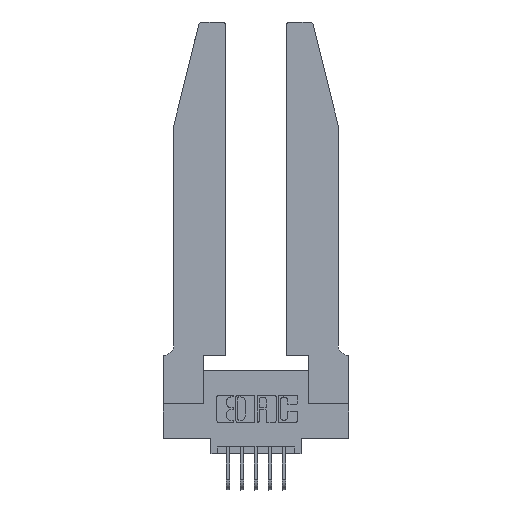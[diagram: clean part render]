
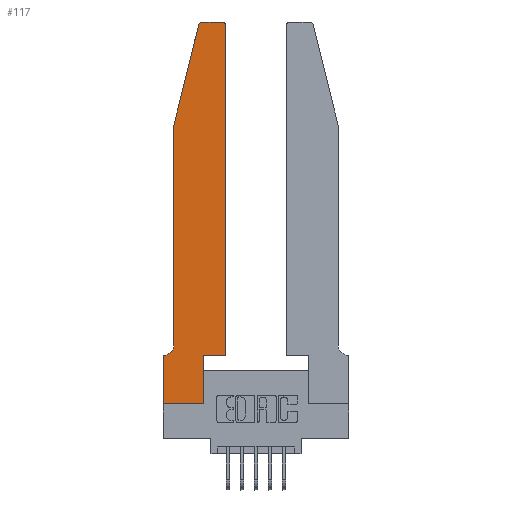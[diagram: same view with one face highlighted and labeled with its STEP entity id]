
A CAD part, top view. The second image highlights one B-rep face of the part: STEP entity #117.
In plain terms, the highlighted planar face has unit normal (0, 0, 1).
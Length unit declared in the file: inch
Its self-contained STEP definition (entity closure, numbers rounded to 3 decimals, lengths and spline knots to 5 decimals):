
#63 = VECTOR ( 'NONE', #1782, 39.37008 ) ;
#117 = ADVANCED_FACE ( 'NONE', ( #862 ), #8695, .T. ) ;
#300 = CARTESIAN_POINT ( 'NONE',  ( 0.4505, 2.72, 0.37 ) ) ;
#314 = EDGE_CURVE ( 'NONE', #7431, #4045, #7570, .T. ) ;
#527 = EDGE_CURVE ( 'NONE', #2413, #6598, #13516, .T. ) ;
#618 = ORIENTED_EDGE ( 'NONE', *, *, #4675, .T. ) ;
#675 = AXIS2_PLACEMENT_3D ( 'NONE', #6815, #3058, #14573 ) ;
#803 = DIRECTION ( 'NONE',  ( 0., -1., 0. ) ) ;
#862 = FACE_OUTER_BOUND ( 'NONE', #14978, .T. ) ;
#1060 = CARTESIAN_POINT ( 'NONE',  ( 0.4205, 2.72, 0.37 ) ) ;
#1276 = LINE ( 'NONE', #15363, #15264 ) ;
#1347 = EDGE_CURVE ( 'NONE', #2260, #3297, #3991, .T. ) ;
#1771 = EDGE_CURVE ( 'NONE', #14939, #13791, #2119, .T. ) ;
#1782 = DIRECTION ( 'NONE',  ( 1., 0., 0. ) ) ;
#2007 = ORIENTED_EDGE ( 'NONE', *, *, #4470, .T. ) ;
#2119 = CIRCLE ( 'NONE', #14043, 0.03 ) ;
#2143 = VECTOR ( 'NONE', #8128, 39.37008 ) ;
#2160 = AXIS2_PLACEMENT_3D ( 'NONE', #6395, #7583, #4897 ) ;
#2260 = VERTEX_POINT ( 'NONE', #5436 ) ;
#2361 = EDGE_CURVE ( 'NONE', #13791, #7431, #9934, .T. ) ;
#2413 = VERTEX_POINT ( 'NONE', #10588 ) ;
#2636 = CARTESIAN_POINT ( 'NONE',  ( 0.2865, 0.35, 0.37 ) ) ;
#3058 = DIRECTION ( 'NONE',  ( 0., 0., -1. ) ) ;
#3066 = CARTESIAN_POINT ( 'NONE',  ( 0.0755, 0.42, 0.37 ) ) ;
#3091 = EDGE_CURVE ( 'NONE', #6598, #2260, #14383, .T. ) ;
#3104 = DIRECTION ( 'NONE',  ( 0., 1., 0. ) ) ;
#3297 = VERTEX_POINT ( 'NONE', #15257 ) ;
#3706 = ORIENTED_EDGE ( 'NONE', *, *, #4528, .T. ) ;
#3991 = LINE ( 'NONE', #11204, #63 ) ;
#4045 = VERTEX_POINT ( 'NONE', #3066 ) ;
#4470 = EDGE_CURVE ( 'NONE', #3297, #11132, #9689, .T. ) ;
#4505 = CARTESIAN_POINT ( 'NONE',  ( 0., 0., 0.37 ) ) ;
#4528 = EDGE_CURVE ( 'NONE', #7789, #14939, #9113, .T. ) ;
#4675 = EDGE_CURVE ( 'NONE', #8454, #6542, #1276, .T. ) ;
#4768 = DIRECTION ( 'NONE',  ( 0., 0., 1. ) ) ;
#4897 = DIRECTION ( 'NONE',  ( 1., 0., 0. ) ) ;
#4969 = VECTOR ( 'NONE', #803, 39.37008 ) ;
#5436 = CARTESIAN_POINT ( 'NONE',  ( 0.2865, 0.35, 0.37 ) ) ;
#5580 = CARTESIAN_POINT ( 'NONE',  ( 0.4205, 2.75, 0.37 ) ) ;
#5615 = CIRCLE ( 'NONE', #13631, 0.03 ) ;
#6296 = ORIENTED_EDGE ( 'NONE', *, *, #10823, .T. ) ;
#6317 = DIRECTION ( 'NONE',  ( 0., 1., 0. ) ) ;
#6344 = CARTESIAN_POINT ( 'NONE',  ( 0.0055, 0.35, 0.37 ) ) ;
#6395 = CARTESIAN_POINT ( 'NONE',  ( 0., 0.35, 0.37 ) ) ;
#6542 = VERTEX_POINT ( 'NONE', #9201 ) ;
#6598 = VERTEX_POINT ( 'NONE', #10381 ) ;
#6815 = CARTESIAN_POINT ( 'NONE',  ( 0.0055, 0.42, 0.37 ) ) ;
#6856 = CARTESIAN_POINT ( 'NONE',  ( 0.4505, 0.35, 0.37 ) ) ;
#7431 = VERTEX_POINT ( 'NONE', #8783 ) ;
#7570 = LINE ( 'NONE', #12738, #4969 ) ;
#7583 = DIRECTION ( 'NONE',  ( 0., 0., 1. ) ) ;
#7699 = CARTESIAN_POINT ( 'NONE',  ( 0.284, 2.72, 0.37 ) ) ;
#7789 = VERTEX_POINT ( 'NONE', #5580 ) ;
#8128 = DIRECTION ( 'NONE',  ( 1., 0., 0. ) ) ;
#8454 = VERTEX_POINT ( 'NONE', #6344 ) ;
#8695 = PLANE ( 'NONE',  #2160 ) ;
#8783 = CARTESIAN_POINT ( 'NONE',  ( 0.0755, 2., 0.37 ) ) ;
#8814 = VECTOR ( 'NONE', #14830, 39.37008 ) ;
#9020 = CARTESIAN_POINT ( 'NONE',  ( 0.284, 2.75, 0.37 ) ) ;
#9113 = LINE ( 'NONE', #12717, #12659 ) ;
#9179 = DIRECTION ( 'NONE',  ( -1., 0., 0. ) ) ;
#9201 = CARTESIAN_POINT ( 'NONE',  ( 0., 0.35, 0.37 ) ) ;
#9348 = DIRECTION ( 'NONE',  ( -0.239, -0.971, 0. ) ) ;
#9364 = VECTOR ( 'NONE', #6317, 39.37008 ) ;
#9533 = EDGE_CURVE ( 'NONE', #11132, #7789, #5615, .T. ) ;
#9562 = DIRECTION ( 'NONE',  ( 1., 0., 0. ) ) ;
#9689 = LINE ( 'NONE', #6856, #12484 ) ;
#9837 = ORIENTED_EDGE ( 'NONE', *, *, #9533, .T. ) ;
#9934 = LINE ( 'NONE', #15337, #15158 ) ;
#9978 = DIRECTION ( 'NONE',  ( 0., 0., 1. ) ) ;
#9984 = ORIENTED_EDGE ( 'NONE', *, *, #12967, .T. ) ;
#10082 = DIRECTION ( 'NONE',  ( 1., 0., 0. ) ) ;
#10261 = ORIENTED_EDGE ( 'NONE', *, *, #2361, .T. ) ;
#10381 = CARTESIAN_POINT ( 'NONE',  ( 0.2865, 0., 0.37 ) ) ;
#10588 = CARTESIAN_POINT ( 'NONE',  ( 0., 0., 0.37 ) ) ;
#10823 = EDGE_CURVE ( 'NONE', #4045, #8454, #12091, .T. ) ;
#11132 = VERTEX_POINT ( 'NONE', #300 ) ;
#11204 = CARTESIAN_POINT ( 'NONE',  ( 0.4505, 0.35, 0.37 ) ) ;
#12091 = CIRCLE ( 'NONE', #675, 0.07 ) ;
#12325 = ORIENTED_EDGE ( 'NONE', *, *, #1347, .T. ) ;
#12484 = VECTOR ( 'NONE', #3104, 39.37008 ) ;
#12556 = ORIENTED_EDGE ( 'NONE', *, *, #314, .T. ) ;
#12659 = VECTOR ( 'NONE', #9179, 39.37008 ) ;
#12717 = CARTESIAN_POINT ( 'NONE',  ( 0.2605, 2.75, 0.37 ) ) ;
#12738 = CARTESIAN_POINT ( 'NONE',  ( 0.0755, 2., 0.37 ) ) ;
#12890 = CARTESIAN_POINT ( 'NONE',  ( 0.25487, 2.72718, 0.37 ) ) ;
#12899 = ORIENTED_EDGE ( 'NONE', *, *, #1771, .T. ) ;
#12967 = EDGE_CURVE ( 'NONE', #6542, #2413, #15330, .T. ) ;
#13038 = ORIENTED_EDGE ( 'NONE', *, *, #3091, .T. ) ;
#13516 = LINE ( 'NONE', #4505, #2143 ) ;
#13628 = CARTESIAN_POINT ( 'NONE',  ( 0., 0., 0.37 ) ) ;
#13631 = AXIS2_PLACEMENT_3D ( 'NONE', #1060, #4768, #9562 ) ;
#13791 = VERTEX_POINT ( 'NONE', #12890 ) ;
#14043 = AXIS2_PLACEMENT_3D ( 'NONE', #7699, #9978, #10082 ) ;
#14233 = DIRECTION ( 'NONE',  ( -1., 0., 0. ) ) ;
#14383 = LINE ( 'NONE', #2636, #9364 ) ;
#14454 = ORIENTED_EDGE ( 'NONE', *, *, #527, .T. ) ;
#14573 = DIRECTION ( 'NONE',  ( -1., 0., 0. ) ) ;
#14830 = DIRECTION ( 'NONE',  ( 0., -1., 0. ) ) ;
#14939 = VERTEX_POINT ( 'NONE', #9020 ) ;
#14978 = EDGE_LOOP ( 'NONE', ( #3706, #12899, #10261, #12556, #6296, #618, #9984, #14454, #13038, #12325, #2007, #9837 ) ) ;
#15158 = VECTOR ( 'NONE', #9348, 39.37008 ) ;
#15257 = CARTESIAN_POINT ( 'NONE',  ( 0.4505, 0.35, 0.37 ) ) ;
#15264 = VECTOR ( 'NONE', #14233, 39.37008 ) ;
#15330 = LINE ( 'NONE', #13628, #8814 ) ;
#15337 = CARTESIAN_POINT ( 'NONE',  ( 0.0755, 2., 0.37 ) ) ;
#15363 = CARTESIAN_POINT ( 'NONE',  ( 0.0755, 0.35, 0.37 ) ) ;
